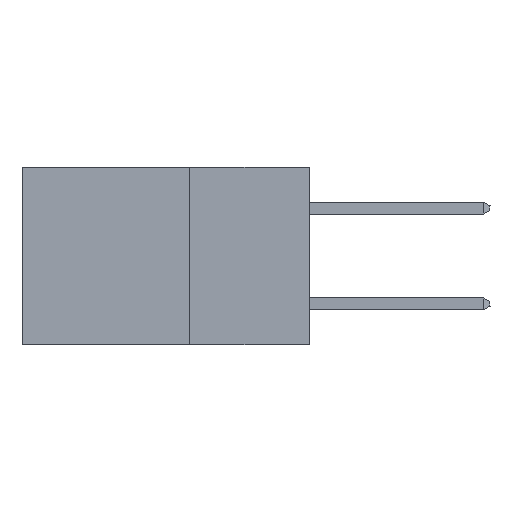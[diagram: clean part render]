
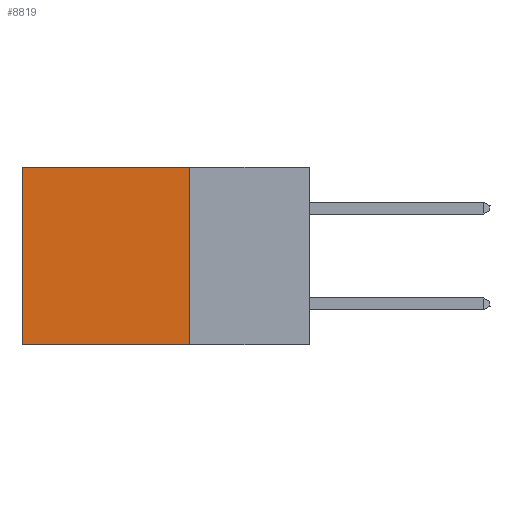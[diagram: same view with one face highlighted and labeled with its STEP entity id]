
A CAD part, left-side view. The second image highlights one B-rep face of the part: STEP entity #8819.
In plain terms, the highlighted planar face has unit normal (-1, 0, 0).
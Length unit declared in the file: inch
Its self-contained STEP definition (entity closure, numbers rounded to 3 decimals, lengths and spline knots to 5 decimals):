
#1921 = EDGE_CURVE ( 'NONE', #12684, #11713, #15597, .T. ) ;
#2116 = EDGE_CURVE ( 'NONE', #11713, #9761, #6151, .T. ) ;
#2479 = VECTOR ( 'NONE', #4002, 39.37008 ) ;
#2852 = VERTEX_POINT ( 'NONE', #4335 ) ;
#3015 = ORIENTED_EDGE ( 'NONE', *, *, #3615, .T. ) ;
#3615 = EDGE_CURVE ( 'NONE', #12684, #2852, #3998, .T. ) ;
#3998 = LINE ( 'NONE', #11009, #14106 ) ;
#4002 = DIRECTION ( 'NONE',  ( 0., 1., 0. ) ) ;
#4335 = CARTESIAN_POINT ( 'NONE',  ( 0.2875, 0.6, 0. ) ) ;
#4500 = LINE ( 'NONE', #9493, #11115 ) ;
#4881 = DIRECTION ( 'NONE',  ( 0., 0., -1. ) ) ;
#5429 = ORIENTED_EDGE ( 'NONE', *, *, #2116, .F. ) ;
#6129 = CARTESIAN_POINT ( 'NONE',  ( 0.2875, 0.25, 0. ) ) ;
#6151 = LINE ( 'NONE', #10544, #2479 ) ;
#6180 = CARTESIAN_POINT ( 'NONE',  ( 0.2875, 0.25, 0. ) ) ;
#6277 = CARTESIAN_POINT ( 'NONE',  ( 0.2875, 0.25, 0. ) ) ;
#6327 = DIRECTION ( 'NONE',  ( 1., 0., 0. ) ) ;
#8094 = EDGE_LOOP ( 'NONE', ( #8430, #5429, #14291, #3015 ) ) ;
#8430 = ORIENTED_EDGE ( 'NONE', *, *, #12349, .T. ) ;
#8497 = CARTESIAN_POINT ( 'NONE',  ( 0.2875, 0.6, -0.37 ) ) ;
#8819 = ADVANCED_FACE ( 'NONE', ( #11441 ), #16740, .F. ) ;
#9493 = CARTESIAN_POINT ( 'NONE',  ( 0.2875, 0.6, 0. ) ) ;
#9761 = VERTEX_POINT ( 'NONE', #8497 ) ;
#10544 = CARTESIAN_POINT ( 'NONE',  ( 0.2875, 0.25, -0.37 ) ) ;
#10802 = DIRECTION ( 'NONE',  ( 0., 0., -1. ) ) ;
#11009 = CARTESIAN_POINT ( 'NONE',  ( 0.2875, 0.25, 0. ) ) ;
#11115 = VECTOR ( 'NONE', #10802, 39.37008 ) ;
#11441 = FACE_OUTER_BOUND ( 'NONE', #8094, .T. ) ;
#11713 = VERTEX_POINT ( 'NONE', #14725 ) ;
#12154 = VECTOR ( 'NONE', #4881, 39.37008 ) ;
#12349 = EDGE_CURVE ( 'NONE', #2852, #9761, #4500, .T. ) ;
#12684 = VERTEX_POINT ( 'NONE', #6129 ) ;
#14106 = VECTOR ( 'NONE', #16215, 39.37008 ) ;
#14291 = ORIENTED_EDGE ( 'NONE', *, *, #1921, .F. ) ;
#14725 = CARTESIAN_POINT ( 'NONE',  ( 0.2875, 0.25, -0.37 ) ) ;
#15502 = DIRECTION ( 'NONE',  ( 0., 0., -1. ) ) ;
#15597 = LINE ( 'NONE', #6180, #12154 ) ;
#16215 = DIRECTION ( 'NONE',  ( 0., 1., 0. ) ) ;
#16618 = AXIS2_PLACEMENT_3D ( 'NONE', #6277, #6327, #15502 ) ;
#16740 = PLANE ( 'NONE',  #16618 ) ;
